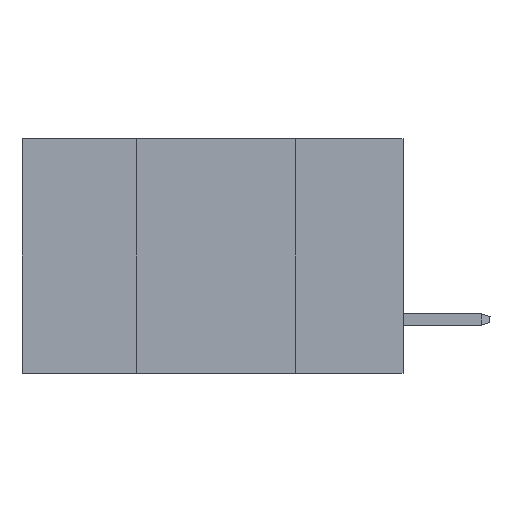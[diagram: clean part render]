
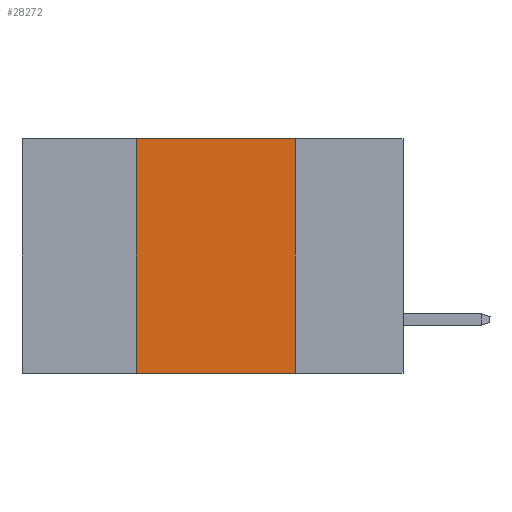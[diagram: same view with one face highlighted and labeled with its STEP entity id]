
A CAD part, left-side view. The second image highlights one B-rep face of the part: STEP entity #28272.
In plain terms, the highlighted planar face has unit normal (-1, 0, 0).
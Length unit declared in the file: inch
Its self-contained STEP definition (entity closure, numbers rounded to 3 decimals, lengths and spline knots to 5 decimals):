
#1835 = LINE ( 'NONE', #21481, #9821 ) ;
#4377 = LINE ( 'NONE', #27480, #39165 ) ;
#5458 = CARTESIAN_POINT ( 'NONE',  ( 0., 0.17, 0. ) ) ;
#5954 = DIRECTION ( 'NONE',  ( 0., 0., -1. ) ) ;
#8324 = VECTOR ( 'NONE', #12234, 39.37008 ) ;
#8836 = DIRECTION ( 'NONE',  ( 0., -1., 0. ) ) ;
#9821 = VECTOR ( 'NONE', #32189, 39.37008 ) ;
#11630 = PLANE ( 'NONE',  #15104 ) ;
#12234 = DIRECTION ( 'NONE',  ( 0., -1., 0. ) ) ;
#12616 = CARTESIAN_POINT ( 'NONE',  ( 0., 0.42, -0.37 ) ) ;
#15104 = AXIS2_PLACEMENT_3D ( 'NONE', #48925, #30994, #15610 ) ;
#15610 = DIRECTION ( 'NONE',  ( 0., 0., -1. ) ) ;
#16789 = ORIENTED_EDGE ( 'NONE', *, *, #18677, .F. ) ;
#18034 = VERTEX_POINT ( 'NONE', #12616 ) ;
#18677 = EDGE_CURVE ( 'NONE', #18034, #33671, #1835, .T. ) ;
#19598 = EDGE_CURVE ( 'NONE', #41460, #23113, #46948, .T. ) ;
#19629 = CARTESIAN_POINT ( 'NONE',  ( 0., 0.17, 0. ) ) ;
#19743 = ORIENTED_EDGE ( 'NONE', *, *, #19598, .F. ) ;
#21481 = CARTESIAN_POINT ( 'NONE',  ( 0., 0.42, 0. ) ) ;
#21661 = EDGE_LOOP ( 'NONE', ( #19743, #33466, #16789, #41549 ) ) ;
#23113 = VERTEX_POINT ( 'NONE', #47555 ) ;
#27480 = CARTESIAN_POINT ( 'NONE',  ( 0., 0.6, -0.37 ) ) ;
#28272 = ADVANCED_FACE ( 'NONE', ( #34508 ), #11630, .F. ) ;
#30362 = EDGE_CURVE ( 'NONE', #33671, #41460, #34391, .T. ) ;
#30994 = DIRECTION ( 'NONE',  ( 1., 0., 0. ) ) ;
#32189 = DIRECTION ( 'NONE',  ( 0., 0., 1. ) ) ;
#33466 = ORIENTED_EDGE ( 'NONE', *, *, #30362, .F. ) ;
#33671 = VERTEX_POINT ( 'NONE', #37508 ) ;
#34391 = LINE ( 'NONE', #34641, #8324 ) ;
#34508 = FACE_OUTER_BOUND ( 'NONE', #21661, .T. ) ;
#34641 = CARTESIAN_POINT ( 'NONE',  ( 0., 0.6, 0. ) ) ;
#36048 = VECTOR ( 'NONE', #5954, 39.37008 ) ;
#37508 = CARTESIAN_POINT ( 'NONE',  ( 0., 0.42, 0. ) ) ;
#39165 = VECTOR ( 'NONE', #8836, 39.37008 ) ;
#41460 = VERTEX_POINT ( 'NONE', #19629 ) ;
#41549 = ORIENTED_EDGE ( 'NONE', *, *, #44264, .T. ) ;
#44264 = EDGE_CURVE ( 'NONE', #18034, #23113, #4377, .T. ) ;
#46948 = LINE ( 'NONE', #5458, #36048 ) ;
#47555 = CARTESIAN_POINT ( 'NONE',  ( 0., 0.17, -0.37 ) ) ;
#48925 = CARTESIAN_POINT ( 'NONE',  ( 0., 0.6, 0. ) ) ;
